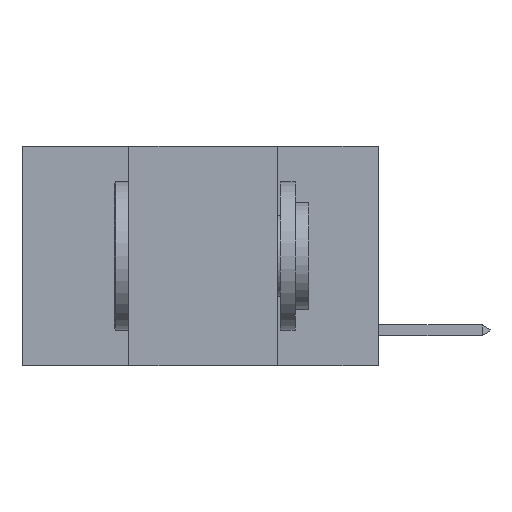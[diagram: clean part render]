
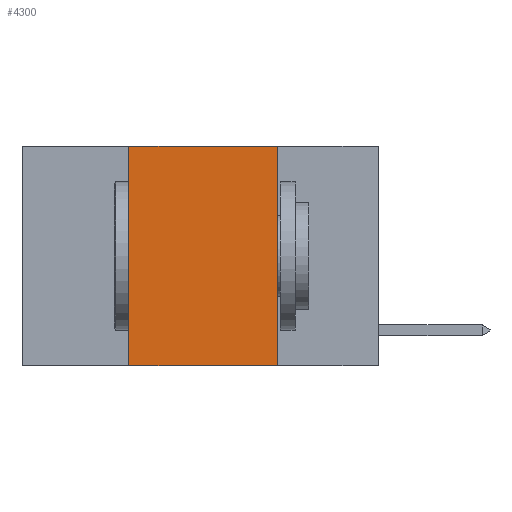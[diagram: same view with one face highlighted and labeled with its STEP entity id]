
A CAD part, left-side view. The second image highlights one B-rep face of the part: STEP entity #4300.
In plain terms, the highlighted planar face has unit normal (-1, 0, 0).
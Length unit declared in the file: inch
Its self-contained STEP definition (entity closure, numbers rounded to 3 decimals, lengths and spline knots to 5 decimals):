
#32 = VECTOR ( 'NONE', #6833, 39.37008 ) ;
#388 = DIRECTION ( 'NONE',  ( 0., 0., 1. ) ) ;
#417 = AXIS2_PLACEMENT_3D ( 'NONE', #8230, #9506, #10780 ) ;
#430 = EDGE_CURVE ( 'NONE', #12844, #3607, #15938, .T. ) ;
#2220 = LINE ( 'NONE', #10197, #7145 ) ;
#2346 = ORIENTED_EDGE ( 'NONE', *, *, #430, .F. ) ;
#3014 = LINE ( 'NONE', #15066, #32 ) ;
#3555 = ORIENTED_EDGE ( 'NONE', *, *, #4817, .F. ) ;
#3607 = VERTEX_POINT ( 'NONE', #13966 ) ;
#4300 = ADVANCED_FACE ( 'NONE', ( #9440 ), #15690, .F. ) ;
#4714 = CARTESIAN_POINT ( 'NONE',  ( 0., 0.42, 0. ) ) ;
#4817 = EDGE_CURVE ( 'NONE', #6716, #12844, #2220, .T. ) ;
#5684 = ORIENTED_EDGE ( 'NONE', *, *, #16205, .F. ) ;
#5934 = VECTOR ( 'NONE', #14635, 39.37008 ) ;
#6493 = ORIENTED_EDGE ( 'NONE', *, *, #12546, .T. ) ;
#6716 = VERTEX_POINT ( 'NONE', #13115 ) ;
#6833 = DIRECTION ( 'NONE',  ( 0., -1., 0. ) ) ;
#7145 = VECTOR ( 'NONE', #388, 39.37008 ) ;
#7788 = LINE ( 'NONE', #13666, #16016 ) ;
#8230 = CARTESIAN_POINT ( 'NONE',  ( 0., 0.6, 0. ) ) ;
#8249 = VERTEX_POINT ( 'NONE', #8794 ) ;
#8720 = DIRECTION ( 'NONE',  ( 0., 0., -1. ) ) ;
#8794 = CARTESIAN_POINT ( 'NONE',  ( 0., 0.17, -0.37 ) ) ;
#9440 = FACE_OUTER_BOUND ( 'NONE', #12102, .T. ) ;
#9506 = DIRECTION ( 'NONE',  ( 1., 0., 0. ) ) ;
#10197 = CARTESIAN_POINT ( 'NONE',  ( 0., 0.42, 0. ) ) ;
#10780 = DIRECTION ( 'NONE',  ( 0., 0., -1. ) ) ;
#12102 = EDGE_LOOP ( 'NONE', ( #5684, #2346, #3555, #6493 ) ) ;
#12546 = EDGE_CURVE ( 'NONE', #6716, #8249, #3014, .T. ) ;
#12844 = VERTEX_POINT ( 'NONE', #4714 ) ;
#13115 = CARTESIAN_POINT ( 'NONE',  ( 0., 0.42, -0.37 ) ) ;
#13666 = CARTESIAN_POINT ( 'NONE',  ( 0., 0.17, 0. ) ) ;
#13966 = CARTESIAN_POINT ( 'NONE',  ( 0., 0.17, 0. ) ) ;
#14382 = CARTESIAN_POINT ( 'NONE',  ( 0., 0.6, 0. ) ) ;
#14635 = DIRECTION ( 'NONE',  ( 0., -1., 0. ) ) ;
#15066 = CARTESIAN_POINT ( 'NONE',  ( 0., 0.6, -0.37 ) ) ;
#15690 = PLANE ( 'NONE',  #417 ) ;
#15938 = LINE ( 'NONE', #14382, #5934 ) ;
#16016 = VECTOR ( 'NONE', #8720, 39.37008 ) ;
#16205 = EDGE_CURVE ( 'NONE', #3607, #8249, #7788, .T. ) ;
